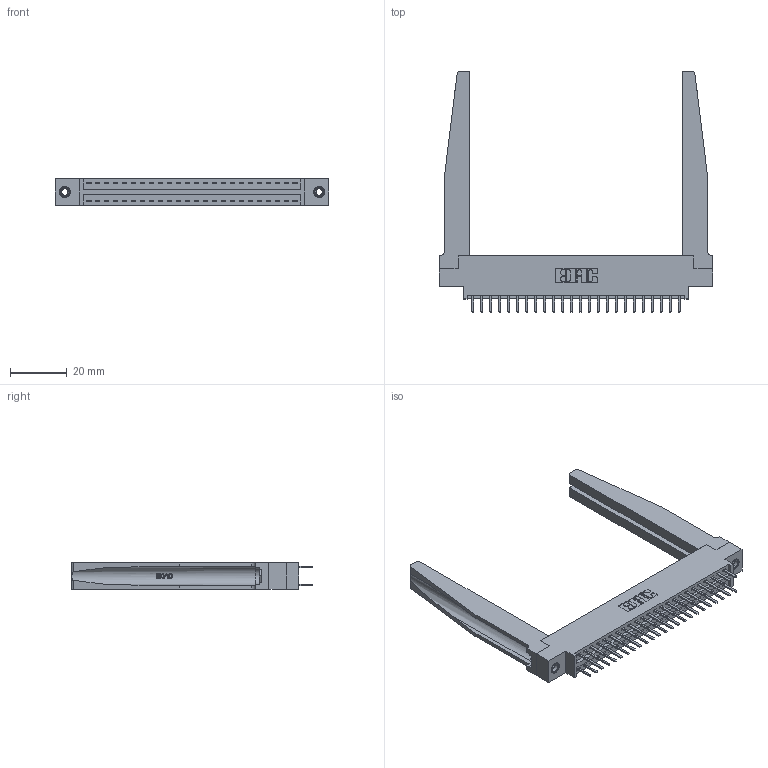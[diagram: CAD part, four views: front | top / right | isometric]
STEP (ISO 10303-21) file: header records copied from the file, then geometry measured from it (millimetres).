
FILE_DESCRIPTION (( 'STEP AP203' ), '1' );
FILE_NAME ('396-048-520-878.STEP', '2019-11-02T06:54:21', ( '' ), ( '' ), 'SwSTEP 2.0', 'SolidWorks 2016', '' );
FILE_SCHEMA (( 'CONFIG_CONTROL_DESIGN' ));
Length unit declared in the file: inch
Products named in the file (5): 346 Part_0.170 Offset - 0.156 Dia-TH; 345-292-001_345-293-120; 346-220-078_345-220-078; 345-250-001_345-250-001-102; 396-048-520-878
Assembly tree (53 placements, depth 2):
  396-048-520-878
    346 Part_0.170 Offset - 0.156 Dia-TH
    345-292-001_345-293-120  x48
    346-220-078_345-220-078  x2
    345-250-001_345-250-001-102  x2
Bounding box: 96.77 x 85.29 x 9.4 mm (x, y, z)
Volume: 16030 mm3; surface area: 18922.4 mm2
Topology: 53 solids, 53 shells, 3048 faces, 8773 edges, 5710 vertices
Faces by surface type: plane 1998, cylinder 998, bspline 36, cone 12, torus 4
Entity records: 23080 total; most frequent: CARTESIAN_POINT 4779, ORIENTED_EDGE 3590, DIRECTION 3237, EDGE_CURVE 1795, LINE 1469, VECTOR 1469, VERTEX_POINT 1188, AXIS2_PLACEMENT_3D 884
